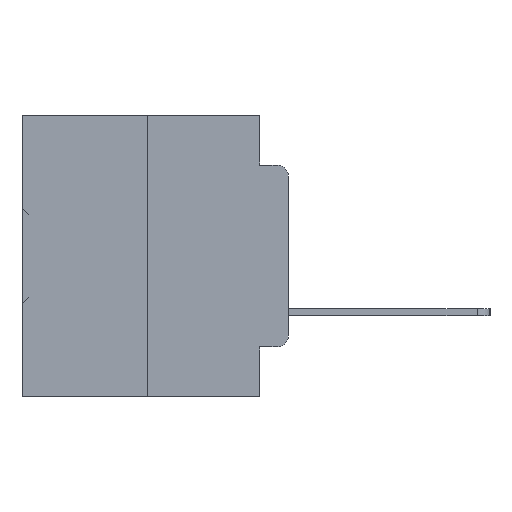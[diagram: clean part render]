
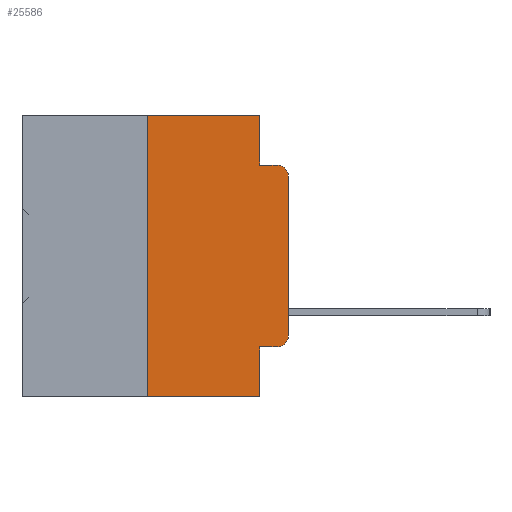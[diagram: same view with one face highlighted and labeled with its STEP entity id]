
A CAD part, left-side view. The second image highlights one B-rep face of the part: STEP entity #25586.
In plain terms, the highlighted planar face has unit normal (-1, 0, 0).
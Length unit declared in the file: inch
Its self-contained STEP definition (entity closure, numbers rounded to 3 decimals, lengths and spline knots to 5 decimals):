
#898 = VECTOR ( 'NONE', #1562, 39.37008 ) ;
#1562 = DIRECTION ( 'NONE',  ( 0., 0., 1. ) ) ;
#1844 = LINE ( 'NONE', #16289, #898 ) ;
#2409 = VECTOR ( 'NONE', #34784, 39.37008 ) ;
#3538 = VERTEX_POINT ( 'NONE', #9654 ) ;
#4007 = VERTEX_POINT ( 'NONE', #17917 ) ;
#4322 = LINE ( 'NONE', #28752, #19047 ) ;
#5547 = DIRECTION ( 'NONE',  ( 0., 0., -1. ) ) ;
#6693 = ORIENTED_EDGE ( 'NONE', *, *, #27597, .F. ) ;
#7330 = VERTEX_POINT ( 'NONE', #28355 ) ;
#7568 = CIRCLE ( 'NONE', #17666, 0.02 ) ;
#7772 = CARTESIAN_POINT ( 'NONE',  ( 0., 0.473, 0. ) ) ;
#7891 = DIRECTION ( 'NONE',  ( 0., 0., -1. ) ) ;
#8240 = CARTESIAN_POINT ( 'NONE',  ( 0., 0.473, 0. ) ) ;
#8480 = CIRCLE ( 'NONE', #19078, 0.02 ) ;
#9654 = CARTESIAN_POINT ( 'NONE',  ( 0., 0.051, -0.4115 ) ) ;
#10080 = EDGE_CURVE ( 'NONE', #34253, #7330, #8480, .T. ) ;
#10487 = CARTESIAN_POINT ( 'NONE',  ( 0., 0.051, -0.5 ) ) ;
#10589 = CARTESIAN_POINT ( 'NONE',  ( 0., 0.02, -0.0885 ) ) ;
#11609 = LINE ( 'NONE', #8240, #17531 ) ;
#11643 = DIRECTION ( 'NONE',  ( 0., -1., 0. ) ) ;
#11897 = CARTESIAN_POINT ( 'NONE',  ( 0., 0.473, -0.5 ) ) ;
#12055 = EDGE_CURVE ( 'NONE', #3538, #34253, #13209, .T. ) ;
#12716 = CARTESIAN_POINT ( 'NONE',  ( 0., 0.02, -0.4115 ) ) ;
#12900 = DIRECTION ( 'NONE',  ( -1., 0., 0. ) ) ;
#13209 = LINE ( 'NONE', #25392, #34238 ) ;
#13624 = DIRECTION ( 'NONE',  ( 1., 0., 0. ) ) ;
#13733 = DIRECTION ( 'NONE',  ( -1., 0., 0. ) ) ;
#14005 = EDGE_CURVE ( 'NONE', #3538, #15539, #4322, .T. ) ;
#14492 = ORIENTED_EDGE ( 'NONE', *, *, #26592, .T. ) ;
#15539 = VERTEX_POINT ( 'NONE', #10487 ) ;
#16289 = CARTESIAN_POINT ( 'NONE',  ( 0., 0., 0. ) ) ;
#16448 = PLANE ( 'NONE',  #24190 ) ;
#16568 = CARTESIAN_POINT ( 'NONE',  ( 0., 0.051, 0. ) ) ;
#17531 = VECTOR ( 'NONE', #26287, 39.37008 ) ;
#17666 = AXIS2_PLACEMENT_3D ( 'NONE', #30925, #13733, #33731 ) ;
#17917 = CARTESIAN_POINT ( 'NONE',  ( 0., 0.051, -0.0885 ) ) ;
#18334 = VECTOR ( 'NONE', #27515, 39.37008 ) ;
#19047 = VECTOR ( 'NONE', #5547, 39.37008 ) ;
#19078 = AXIS2_PLACEMENT_3D ( 'NONE', #30109, #12900, #32938 ) ;
#20245 = LINE ( 'NONE', #28895, #34456 ) ;
#20285 = EDGE_LOOP ( 'NONE', ( #33162, #35815, #34972, #36756, #6693, #31515, #14492, #36289, #31489, #30168 ) ) ;
#20962 = VERTEX_POINT ( 'NONE', #22439 ) ;
#21887 = VERTEX_POINT ( 'NONE', #35214 ) ;
#22439 = CARTESIAN_POINT ( 'NONE',  ( 0., 0.25, -0.5 ) ) ;
#22707 = CARTESIAN_POINT ( 'NONE',  ( 0., 0.25, 0. ) ) ;
#23650 = EDGE_CURVE ( 'NONE', #20962, #26722, #36112, .T. ) ;
#24190 = AXIS2_PLACEMENT_3D ( 'NONE', #7772, #13624, #33636 ) ;
#24599 = CARTESIAN_POINT ( 'NONE',  ( 0., 0.25, 0. ) ) ;
#25392 = CARTESIAN_POINT ( 'NONE',  ( 0., 0.051, -0.4115 ) ) ;
#25586 = ADVANCED_FACE ( 'NONE', ( #31061 ), #16448, .F. ) ;
#25630 = EDGE_CURVE ( 'NONE', #32267, #4007, #30152, .T. ) ;
#26287 = DIRECTION ( 'NONE',  ( 0., -1., 0. ) ) ;
#26592 = EDGE_CURVE ( 'NONE', #20962, #15539, #30597, .T. ) ;
#26722 = VERTEX_POINT ( 'NONE', #22707 ) ;
#27515 = DIRECTION ( 'NONE',  ( 0., 0., 1. ) ) ;
#27544 = EDGE_CURVE ( 'NONE', #4007, #28951, #20245, .T. ) ;
#27597 = EDGE_CURVE ( 'NONE', #26722, #32267, #11609, .T. ) ;
#28247 = DIRECTION ( 'NONE',  ( 0., -1., 0. ) ) ;
#28355 = CARTESIAN_POINT ( 'NONE',  ( 0., 0., -0.3915 ) ) ;
#28752 = CARTESIAN_POINT ( 'NONE',  ( 0., 0.051, 0. ) ) ;
#28895 = CARTESIAN_POINT ( 'NONE',  ( 0., 0.051, -0.0885 ) ) ;
#28951 = VERTEX_POINT ( 'NONE', #10589 ) ;
#29258 = VECTOR ( 'NONE', #7891, 39.37008 ) ;
#30109 = CARTESIAN_POINT ( 'NONE',  ( 0., 0.02, -0.3915 ) ) ;
#30152 = LINE ( 'NONE', #16568, #29258 ) ;
#30168 = ORIENTED_EDGE ( 'NONE', *, *, #10080, .T. ) ;
#30397 = CARTESIAN_POINT ( 'NONE',  ( 0., 0.051, 0. ) ) ;
#30597 = LINE ( 'NONE', #11897, #2409 ) ;
#30925 = CARTESIAN_POINT ( 'NONE',  ( 0., 0.02, -0.1085 ) ) ;
#31061 = FACE_OUTER_BOUND ( 'NONE', #20285, .T. ) ;
#31489 = ORIENTED_EDGE ( 'NONE', *, *, #12055, .T. ) ;
#31515 = ORIENTED_EDGE ( 'NONE', *, *, #23650, .F. ) ;
#32267 = VERTEX_POINT ( 'NONE', #30397 ) ;
#32938 = DIRECTION ( 'NONE',  ( 0., 0., -1. ) ) ;
#33162 = ORIENTED_EDGE ( 'NONE', *, *, #36943, .T. ) ;
#33636 = DIRECTION ( 'NONE',  ( 0., 0., -1. ) ) ;
#33731 = DIRECTION ( 'NONE',  ( 0., 0., -1. ) ) ;
#34238 = VECTOR ( 'NONE', #28247, 39.37008 ) ;
#34253 = VERTEX_POINT ( 'NONE', #12716 ) ;
#34456 = VECTOR ( 'NONE', #11643, 39.37008 ) ;
#34784 = DIRECTION ( 'NONE',  ( 0., -1., 0. ) ) ;
#34972 = ORIENTED_EDGE ( 'NONE', *, *, #27544, .F. ) ;
#35041 = EDGE_CURVE ( 'NONE', #21887, #28951, #7568, .T. ) ;
#35214 = CARTESIAN_POINT ( 'NONE',  ( 0., 0., -0.1085 ) ) ;
#35815 = ORIENTED_EDGE ( 'NONE', *, *, #35041, .T. ) ;
#36112 = LINE ( 'NONE', #24599, #18334 ) ;
#36289 = ORIENTED_EDGE ( 'NONE', *, *, #14005, .F. ) ;
#36756 = ORIENTED_EDGE ( 'NONE', *, *, #25630, .F. ) ;
#36943 = EDGE_CURVE ( 'NONE', #7330, #21887, #1844, .T. ) ;
